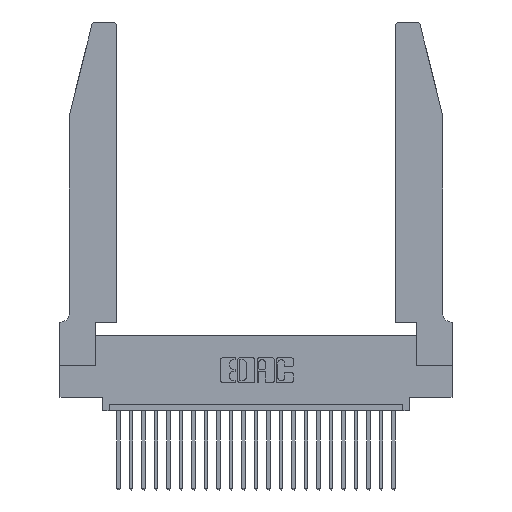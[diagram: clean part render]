
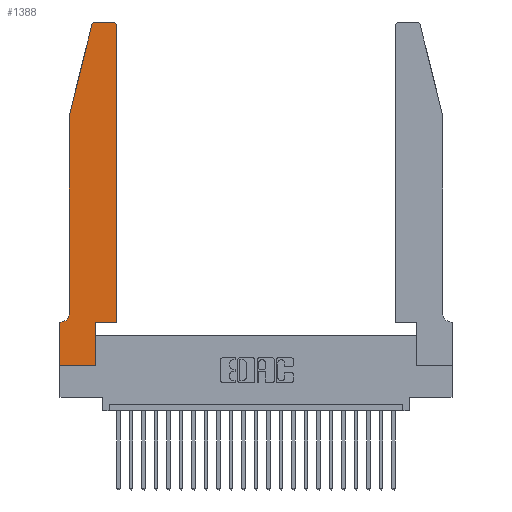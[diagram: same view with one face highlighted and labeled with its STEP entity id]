
A CAD part, top view. The second image highlights one B-rep face of the part: STEP entity #1388.
In plain terms, the highlighted planar face has unit normal (0, 0, 1).
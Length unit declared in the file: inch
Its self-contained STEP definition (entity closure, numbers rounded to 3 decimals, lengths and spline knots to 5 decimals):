
#108 = DIRECTION ( 'NONE',  ( -1., 0., 0. ) ) ;
#145 = EDGE_CURVE ( 'NONE', #9714, #8591, #14562, .T. ) ;
#433 = ORIENTED_EDGE ( 'NONE', *, *, #770, .T. ) ;
#770 = EDGE_CURVE ( 'NONE', #9061, #15296, #13897, .T. ) ;
#793 = CARTESIAN_POINT ( 'NONE',  ( 0.0755, 0.42, 0.37 ) ) ;
#795 = DIRECTION ( 'NONE',  ( 1., 0., 0. ) ) ;
#1154 = EDGE_CURVE ( 'NONE', #15630, #8247, #5244, .T. ) ;
#1388 = ADVANCED_FACE ( 'NONE', ( #2527 ), #17950, .T. ) ;
#1609 = VERTEX_POINT ( 'NONE', #1856 ) ;
#1856 = CARTESIAN_POINT ( 'NONE',  ( 0.4205, 2.75, 0.37 ) ) ;
#2102 = LINE ( 'NONE', #21301, #6892 ) ;
#2207 = VERTEX_POINT ( 'NONE', #22591 ) ;
#2527 = FACE_OUTER_BOUND ( 'NONE', #10941, .T. ) ;
#2773 = DIRECTION ( 'NONE',  ( 1., 0., 0. ) ) ;
#3148 = DIRECTION ( 'NONE',  ( 0., 0., 1. ) ) ;
#3504 = EDGE_CURVE ( 'NONE', #8591, #2207, #2102, .T. ) ;
#3916 = CARTESIAN_POINT ( 'NONE',  ( 0.284, 2.75, 0.37 ) ) ;
#4194 = ORIENTED_EDGE ( 'NONE', *, *, #8749, .T. ) ;
#4671 = DIRECTION ( 'NONE',  ( 0., -1., 0. ) ) ;
#4674 = DIRECTION ( 'NONE',  ( 0., 1., 0. ) ) ;
#4708 = VERTEX_POINT ( 'NONE', #9551 ) ;
#4755 = DIRECTION ( 'NONE',  ( 0., 0., -1. ) ) ;
#5009 = ORIENTED_EDGE ( 'NONE', *, *, #8762, .T. ) ;
#5021 = VECTOR ( 'NONE', #19438, 39.37008 ) ;
#5217 = LINE ( 'NONE', #21836, #14770 ) ;
#5244 = LINE ( 'NONE', #21455, #6722 ) ;
#5245 = AXIS2_PLACEMENT_3D ( 'NONE', #6783, #4755, #8841 ) ;
#5861 = VECTOR ( 'NONE', #108, 39.37008 ) ;
#6041 = CARTESIAN_POINT ( 'NONE',  ( 0.2605, 2.75, 0.37 ) ) ;
#6219 = LINE ( 'NONE', #23907, #11285 ) ;
#6518 = CARTESIAN_POINT ( 'NONE',  ( 0.0055, 0.35, 0.37 ) ) ;
#6634 = AXIS2_PLACEMENT_3D ( 'NONE', #6977, #3148, #24443 ) ;
#6722 = VECTOR ( 'NONE', #22265, 39.37008 ) ;
#6783 = CARTESIAN_POINT ( 'NONE',  ( 0.0055, 0.42, 0.37 ) ) ;
#6892 = VECTOR ( 'NONE', #13640, 39.37008 ) ;
#6977 = CARTESIAN_POINT ( 'NONE',  ( 0.284, 2.72, 0.37 ) ) ;
#7813 = CARTESIAN_POINT ( 'NONE',  ( 0.0755, 0.35, 0.37 ) ) ;
#8007 = LINE ( 'NONE', #6041, #5021 ) ;
#8243 = CARTESIAN_POINT ( 'NONE',  ( 0., 0., 0.37 ) ) ;
#8247 = VERTEX_POINT ( 'NONE', #793 ) ;
#8438 = DIRECTION ( 'NONE',  ( -0.239, -0.971, 0. ) ) ;
#8554 = CARTESIAN_POINT ( 'NONE',  ( 0., 0.35, 0.37 ) ) ;
#8591 = VERTEX_POINT ( 'NONE', #16508 ) ;
#8749 = EDGE_CURVE ( 'NONE', #15296, #18729, #6219, .T. ) ;
#8762 = EDGE_CURVE ( 'NONE', #8247, #9061, #21794, .T. ) ;
#8841 = DIRECTION ( 'NONE',  ( -1., 0., 0. ) ) ;
#8862 = LINE ( 'NONE', #18152, #21758 ) ;
#9061 = VERTEX_POINT ( 'NONE', #6518 ) ;
#9383 = DIRECTION ( 'NONE',  ( 1., 0., 0. ) ) ;
#9551 = CARTESIAN_POINT ( 'NONE',  ( 0.2865, 0., 0.37 ) ) ;
#9684 = AXIS2_PLACEMENT_3D ( 'NONE', #17533, #24550, #9383 ) ;
#9714 = VERTEX_POINT ( 'NONE', #12799 ) ;
#10566 = VERTEX_POINT ( 'NONE', #20269 ) ;
#10941 = EDGE_LOOP ( 'NONE', ( #15148, #12027, #11012, #14080, #5009, #433, #4194, #15786, #14159, #15461, #13278, #11247 ) ) ;
#11012 = ORIENTED_EDGE ( 'NONE', *, *, #17143, .T. ) ;
#11247 = ORIENTED_EDGE ( 'NONE', *, *, #18885, .T. ) ;
#11285 = VECTOR ( 'NONE', #4671, 39.37008 ) ;
#12027 = ORIENTED_EDGE ( 'NONE', *, *, #16763, .T. ) ;
#12615 = CARTESIAN_POINT ( 'NONE',  ( 0.4505, 0.35, 0.37 ) ) ;
#12799 = CARTESIAN_POINT ( 'NONE',  ( 0.2865, 0.35, 0.37 ) ) ;
#13278 = ORIENTED_EDGE ( 'NONE', *, *, #3504, .T. ) ;
#13547 = LINE ( 'NONE', #16154, #15078 ) ;
#13580 = EDGE_CURVE ( 'NONE', #1609, #15821, #8007, .T. ) ;
#13640 = DIRECTION ( 'NONE',  ( 0., 1., 0. ) ) ;
#13897 = LINE ( 'NONE', #7813, #5861 ) ;
#14080 = ORIENTED_EDGE ( 'NONE', *, *, #1154, .T. ) ;
#14159 = ORIENTED_EDGE ( 'NONE', *, *, #22142, .T. ) ;
#14562 = LINE ( 'NONE', #12615, #19093 ) ;
#14770 = VECTOR ( 'NONE', #2773, 39.37008 ) ;
#15078 = VECTOR ( 'NONE', #8438, 39.37008 ) ;
#15143 = DIRECTION ( 'NONE',  ( 1., 0., 0. ) ) ;
#15148 = ORIENTED_EDGE ( 'NONE', *, *, #13580, .T. ) ;
#15296 = VERTEX_POINT ( 'NONE', #15556 ) ;
#15461 = ORIENTED_EDGE ( 'NONE', *, *, #145, .T. ) ;
#15556 = CARTESIAN_POINT ( 'NONE',  ( 0., 0.35, 0.37 ) ) ;
#15630 = VERTEX_POINT ( 'NONE', #24161 ) ;
#15786 = ORIENTED_EDGE ( 'NONE', *, *, #17190, .T. ) ;
#15821 = VERTEX_POINT ( 'NONE', #3916 ) ;
#16154 = CARTESIAN_POINT ( 'NONE',  ( 0.0755, 2., 0.37 ) ) ;
#16508 = CARTESIAN_POINT ( 'NONE',  ( 0.4505, 0.35, 0.37 ) ) ;
#16763 = EDGE_CURVE ( 'NONE', #15821, #10566, #21386, .T. ) ;
#17143 = EDGE_CURVE ( 'NONE', #10566, #15630, #13547, .T. ) ;
#17190 = EDGE_CURVE ( 'NONE', #18729, #4708, #5217, .T. ) ;
#17533 = CARTESIAN_POINT ( 'NONE',  ( 0.4205, 2.72, 0.37 ) ) ;
#17950 = PLANE ( 'NONE',  #20544 ) ;
#18152 = CARTESIAN_POINT ( 'NONE',  ( 0.2865, 0.35, 0.37 ) ) ;
#18632 = CIRCLE ( 'NONE', #9684, 0.03 ) ;
#18729 = VERTEX_POINT ( 'NONE', #8243 ) ;
#18885 = EDGE_CURVE ( 'NONE', #2207, #1609, #18632, .T. ) ;
#19093 = VECTOR ( 'NONE', #15143, 39.37008 ) ;
#19438 = DIRECTION ( 'NONE',  ( -1., 0., 0. ) ) ;
#20269 = CARTESIAN_POINT ( 'NONE',  ( 0.25487, 2.72718, 0.37 ) ) ;
#20544 = AXIS2_PLACEMENT_3D ( 'NONE', #8554, #21960, #795 ) ;
#21301 = CARTESIAN_POINT ( 'NONE',  ( 0.4505, 0.35, 0.37 ) ) ;
#21386 = CIRCLE ( 'NONE', #6634, 0.03 ) ;
#21455 = CARTESIAN_POINT ( 'NONE',  ( 0.0755, 2., 0.37 ) ) ;
#21758 = VECTOR ( 'NONE', #4674, 39.37008 ) ;
#21794 = CIRCLE ( 'NONE', #5245, 0.07 ) ;
#21836 = CARTESIAN_POINT ( 'NONE',  ( 0., 0., 0.37 ) ) ;
#21960 = DIRECTION ( 'NONE',  ( 0., 0., 1. ) ) ;
#22142 = EDGE_CURVE ( 'NONE', #4708, #9714, #8862, .T. ) ;
#22265 = DIRECTION ( 'NONE',  ( 0., -1., 0. ) ) ;
#22591 = CARTESIAN_POINT ( 'NONE',  ( 0.4505, 2.72, 0.37 ) ) ;
#23907 = CARTESIAN_POINT ( 'NONE',  ( 0., 0., 0.37 ) ) ;
#24161 = CARTESIAN_POINT ( 'NONE',  ( 0.0755, 2., 0.37 ) ) ;
#24443 = DIRECTION ( 'NONE',  ( 1., 0., 0. ) ) ;
#24550 = DIRECTION ( 'NONE',  ( 0., 0., 1. ) ) ;
